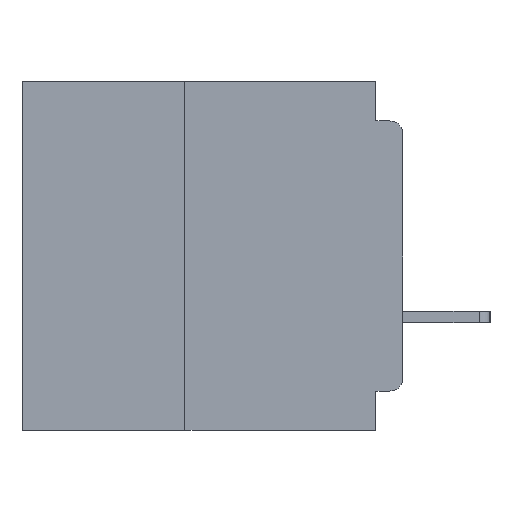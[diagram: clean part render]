
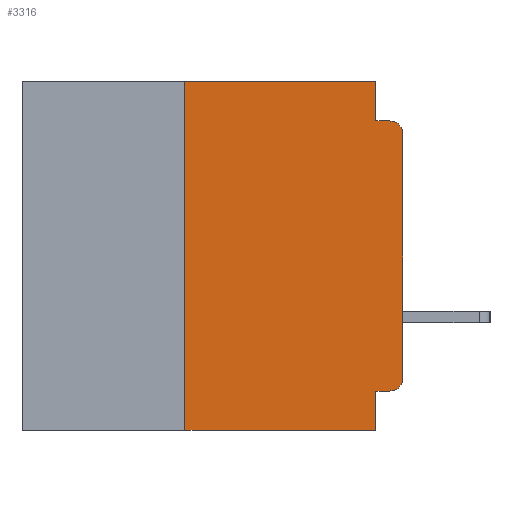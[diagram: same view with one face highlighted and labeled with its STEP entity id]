
A CAD part, left-side view. The second image highlights one B-rep face of the part: STEP entity #3316.
In plain terms, the highlighted planar face has unit normal (-1, 0, 0).
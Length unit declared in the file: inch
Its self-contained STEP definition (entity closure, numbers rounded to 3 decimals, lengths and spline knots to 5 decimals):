
#504 = FACE_OUTER_BOUND ( 'NONE', #11405, .T. ) ;
#553 = CARTESIAN_POINT ( 'NONE',  ( 0., 0., -0.34 ) ) ;
#1249 = VECTOR ( 'NONE', #28576, 39.37008 ) ;
#1936 = ORIENTED_EDGE ( 'NONE', *, *, #19699, .F. ) ;
#2252 = VECTOR ( 'NONE', #16960, 39.37008 ) ;
#2305 = ORIENTED_EDGE ( 'NONE', *, *, #19803, .F. ) ;
#3316 = ADVANCED_FACE ( 'NONE', ( #504 ), #46862, .F. ) ;
#3484 = LINE ( 'NONE', #41605, #26008 ) ;
#3775 = LINE ( 'NONE', #26596, #2252 ) ;
#6984 = CARTESIAN_POINT ( 'NONE',  ( 0., 0.031, 0. ) ) ;
#7245 = DIRECTION ( 'NONE',  ( 0., -1., 0. ) ) ;
#8143 = EDGE_CURVE ( 'NONE', #39596, #20853, #44240, .T. ) ;
#8560 = LINE ( 'NONE', #18278, #45261 ) ;
#9456 = ORIENTED_EDGE ( 'NONE', *, *, #8143, .T. ) ;
#10262 = EDGE_CURVE ( 'NONE', #35962, #16307, #3775, .T. ) ;
#11405 = EDGE_LOOP ( 'NONE', ( #41243, #60257, #2305, #28094, #51576, #1936, #55288, #32184, #26097, #9456 ) ) ;
#12235 = DIRECTION ( 'NONE',  ( 0., 0., 1. ) ) ;
#16307 = VERTEX_POINT ( 'NONE', #6984 ) ;
#16722 = AXIS2_PLACEMENT_3D ( 'NONE', #51332, #22727, #56070 ) ;
#16960 = DIRECTION ( 'NONE',  ( 0., -1., 0. ) ) ;
#17268 = DIRECTION ( 'NONE',  ( 0., 0., -1. ) ) ;
#17809 = EDGE_CURVE ( 'NONE', #61248, #57914, #34533, .T. ) ;
#18222 = DIRECTION ( 'NONE',  ( 1., 0., 0. ) ) ;
#18278 = CARTESIAN_POINT ( 'NONE',  ( 0., 0.031, -0.4 ) ) ;
#19516 = CARTESIAN_POINT ( 'NONE',  ( 0., 0.015, -0.34 ) ) ;
#19699 = EDGE_CURVE ( 'NONE', #47878, #35962, #26851, .T. ) ;
#19803 = EDGE_CURVE ( 'NONE', #47935, #57914, #44755, .T. ) ;
#20853 = VERTEX_POINT ( 'NONE', #553 ) ;
#21630 = LINE ( 'NONE', #29714, #58176 ) ;
#22727 = DIRECTION ( 'NONE',  ( -1., 0., 0. ) ) ;
#22930 = EDGE_CURVE ( 'NONE', #16307, #47935, #60369, .T. ) ;
#23831 = CARTESIAN_POINT ( 'NONE',  ( 0., 0.015, -0.045 ) ) ;
#24354 = DIRECTION ( 'NONE',  ( 0., 0., -1. ) ) ;
#26008 = VECTOR ( 'NONE', #32186, 39.37008 ) ;
#26097 = ORIENTED_EDGE ( 'NONE', *, *, #40248, .F. ) ;
#26596 = CARTESIAN_POINT ( 'NONE',  ( 0., 0.437, 0. ) ) ;
#26851 = LINE ( 'NONE', #38217, #1249 ) ;
#28094 = ORIENTED_EDGE ( 'NONE', *, *, #22930, .F. ) ;
#28576 = DIRECTION ( 'NONE',  ( 0., 0., 1. ) ) ;
#29377 = CARTESIAN_POINT ( 'NONE',  ( 0., 0.031, -0.045 ) ) ;
#29714 = CARTESIAN_POINT ( 'NONE',  ( 0., 0.437, -0.4 ) ) ;
#32184 = ORIENTED_EDGE ( 'NONE', *, *, #56080, .F. ) ;
#32186 = DIRECTION ( 'NONE',  ( 0., 1., 0. ) ) ;
#34533 = CIRCLE ( 'NONE', #16722, 0.015 ) ;
#34725 = CARTESIAN_POINT ( 'NONE',  ( 0., 0.015, -0.355 ) ) ;
#34878 = VECTOR ( 'NONE', #12235, 39.37008 ) ;
#35962 = VERTEX_POINT ( 'NONE', #59001 ) ;
#35975 = CARTESIAN_POINT ( 'NONE',  ( 0., 0., -0.045 ) ) ;
#36141 = CARTESIAN_POINT ( 'NONE',  ( 0., 0., 0. ) ) ;
#37176 = AXIS2_PLACEMENT_3D ( 'NONE', #19516, #52923, #24354 ) ;
#37277 = CARTESIAN_POINT ( 'NONE',  ( 0., 0.437, 0. ) ) ;
#37302 = VERTEX_POINT ( 'NONE', #44839 ) ;
#37904 = AXIS2_PLACEMENT_3D ( 'NONE', #37277, #18222, #51630 ) ;
#38217 = CARTESIAN_POINT ( 'NONE',  ( 0., 0.25, -0.4 ) ) ;
#39596 = VERTEX_POINT ( 'NONE', #34725 ) ;
#40248 = EDGE_CURVE ( 'NONE', #39596, #54225, #3484, .T. ) ;
#41243 = ORIENTED_EDGE ( 'NONE', *, *, #61334, .T. ) ;
#41605 = CARTESIAN_POINT ( 'NONE',  ( 0., 0., -0.355 ) ) ;
#43209 = CARTESIAN_POINT ( 'NONE',  ( 0., 0.25, -0.4 ) ) ;
#44136 = DIRECTION ( 'NONE',  ( 0., -1., 0. ) ) ;
#44240 = CIRCLE ( 'NONE', #37176, 0.015 ) ;
#44755 = LINE ( 'NONE', #35975, #47743 ) ;
#44839 = CARTESIAN_POINT ( 'NONE',  ( 0., 0.031, -0.4 ) ) ;
#45261 = VECTOR ( 'NONE', #57695, 39.37008 ) ;
#46862 = PLANE ( 'NONE',  #37904 ) ;
#47743 = VECTOR ( 'NONE', #7245, 39.37008 ) ;
#47878 = VERTEX_POINT ( 'NONE', #43209 ) ;
#47935 = VERTEX_POINT ( 'NONE', #29377 ) ;
#49497 = CARTESIAN_POINT ( 'NONE',  ( 0., 0., -0.06 ) ) ;
#50705 = CARTESIAN_POINT ( 'NONE',  ( 0., 0.031, 0. ) ) ;
#51332 = CARTESIAN_POINT ( 'NONE',  ( 0., 0.015, -0.06 ) ) ;
#51576 = ORIENTED_EDGE ( 'NONE', *, *, #10262, .F. ) ;
#51630 = DIRECTION ( 'NONE',  ( 0., 0., -1. ) ) ;
#52312 = CARTESIAN_POINT ( 'NONE',  ( 0., 0.031, -0.355 ) ) ;
#52923 = DIRECTION ( 'NONE',  ( -1., 0., 0. ) ) ;
#54225 = VERTEX_POINT ( 'NONE', #52312 ) ;
#55288 = ORIENTED_EDGE ( 'NONE', *, *, #59240, .T. ) ;
#56070 = DIRECTION ( 'NONE',  ( 0., 0., -1. ) ) ;
#56080 = EDGE_CURVE ( 'NONE', #54225, #37302, #8560, .T. ) ;
#57695 = DIRECTION ( 'NONE',  ( 0., 0., -1. ) ) ;
#57914 = VERTEX_POINT ( 'NONE', #23831 ) ;
#58176 = VECTOR ( 'NONE', #44136, 39.37008 ) ;
#58860 = VECTOR ( 'NONE', #17268, 39.37008 ) ;
#59001 = CARTESIAN_POINT ( 'NONE',  ( 0., 0.25, 0. ) ) ;
#59240 = EDGE_CURVE ( 'NONE', #47878, #37302, #21630, .T. ) ;
#60222 = LINE ( 'NONE', #36141, #34878 ) ;
#60257 = ORIENTED_EDGE ( 'NONE', *, *, #17809, .T. ) ;
#60369 = LINE ( 'NONE', #50705, #58860 ) ;
#61248 = VERTEX_POINT ( 'NONE', #49497 ) ;
#61334 = EDGE_CURVE ( 'NONE', #20853, #61248, #60222, .T. ) ;
